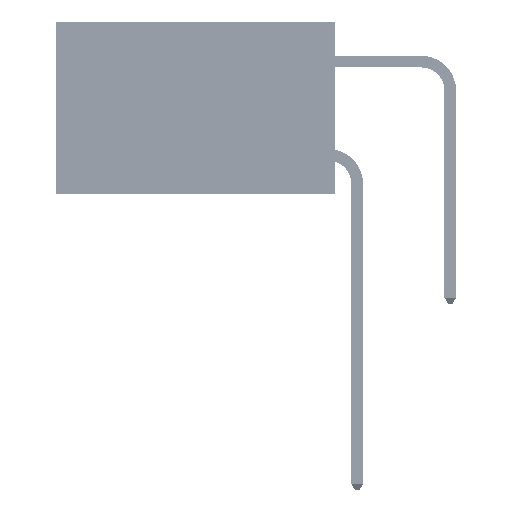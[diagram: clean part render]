
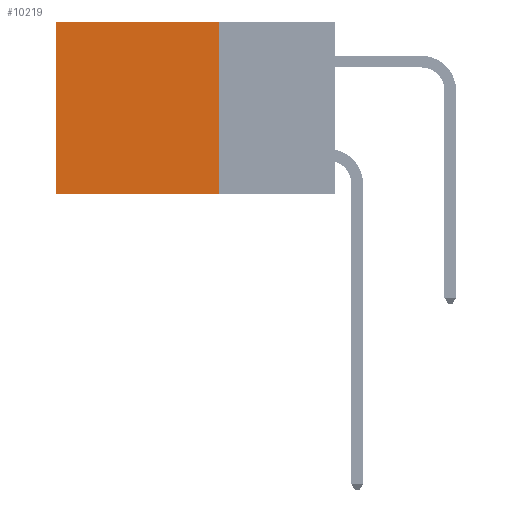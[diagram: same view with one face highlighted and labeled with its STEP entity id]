
A CAD part, left-side view. The second image highlights one B-rep face of the part: STEP entity #10219.
In plain terms, the highlighted planar face has unit normal (-1, 0, 0).
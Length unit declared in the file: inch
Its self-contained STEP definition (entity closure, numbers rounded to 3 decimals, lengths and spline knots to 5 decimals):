
#306 = EDGE_CURVE ( 'NONE', #21380, #44522, #39304, .T. ) ;
#479 = ORIENTED_EDGE ( 'NONE', *, *, #41265, .F. ) ;
#1109 = FACE_OUTER_BOUND ( 'NONE', #28974, .T. ) ;
#1166 = DIRECTION ( 'NONE',  ( 0., 1., 0. ) ) ;
#1181 = DIRECTION ( 'NONE',  ( 0., 0., -1. ) ) ;
#2217 = VERTEX_POINT ( 'NONE', #43689 ) ;
#2546 = ORIENTED_EDGE ( 'NONE', *, *, #37306, .T. ) ;
#2692 = LINE ( 'NONE', #6507, #46127 ) ;
#6507 = CARTESIAN_POINT ( 'NONE',  ( 0.2875, 0.25, 0. ) ) ;
#9168 = LINE ( 'NONE', #25359, #21135 ) ;
#9300 = VERTEX_POINT ( 'NONE', #23185 ) ;
#10130 = AXIS2_PLACEMENT_3D ( 'NONE', #14065, #33567, #29526 ) ;
#10219 = ADVANCED_FACE ( 'NONE', ( #1109 ), #17941, .F. ) ;
#12872 = VECTOR ( 'NONE', #1166, 39.37008 ) ;
#13050 = ORIENTED_EDGE ( 'NONE', *, *, #306, .F. ) ;
#14065 = CARTESIAN_POINT ( 'NONE',  ( 0.2875, 0.25, 0. ) ) ;
#17941 = PLANE ( 'NONE',  #10130 ) ;
#21135 = VECTOR ( 'NONE', #1181, 39.37008 ) ;
#21380 = VERTEX_POINT ( 'NONE', #38142 ) ;
#23185 = CARTESIAN_POINT ( 'NONE',  ( 0.2875, 0.25, 0. ) ) ;
#25359 = CARTESIAN_POINT ( 'NONE',  ( 0.2875, 0.6, 0. ) ) ;
#26522 = EDGE_CURVE ( 'NONE', #9300, #2217, #39815, .T. ) ;
#28313 = ORIENTED_EDGE ( 'NONE', *, *, #26522, .T. ) ;
#28974 = EDGE_LOOP ( 'NONE', ( #2546, #13050, #479, #28313 ) ) ;
#29526 = DIRECTION ( 'NONE',  ( 0., 0., -1. ) ) ;
#33567 = DIRECTION ( 'NONE',  ( 1., 0., 0. ) ) ;
#33756 = CARTESIAN_POINT ( 'NONE',  ( 0.2875, 0.25, -0.37 ) ) ;
#37306 = EDGE_CURVE ( 'NONE', #2217, #44522, #9168, .T. ) ;
#38142 = CARTESIAN_POINT ( 'NONE',  ( 0.2875, 0.25, -0.37 ) ) ;
#39048 = DIRECTION ( 'NONE',  ( 0., 0., -1. ) ) ;
#39304 = LINE ( 'NONE', #33756, #12872 ) ;
#39815 = LINE ( 'NONE', #41617, #45460 ) ;
#41265 = EDGE_CURVE ( 'NONE', #9300, #21380, #2692, .T. ) ;
#41617 = CARTESIAN_POINT ( 'NONE',  ( 0.2875, 0.25, 0. ) ) ;
#43689 = CARTESIAN_POINT ( 'NONE',  ( 0.2875, 0.6, 0. ) ) ;
#44522 = VERTEX_POINT ( 'NONE', #45702 ) ;
#45320 = DIRECTION ( 'NONE',  ( 0., 1., 0. ) ) ;
#45460 = VECTOR ( 'NONE', #45320, 39.37008 ) ;
#45702 = CARTESIAN_POINT ( 'NONE',  ( 0.2875, 0.6, -0.37 ) ) ;
#46127 = VECTOR ( 'NONE', #39048, 39.37008 ) ;
